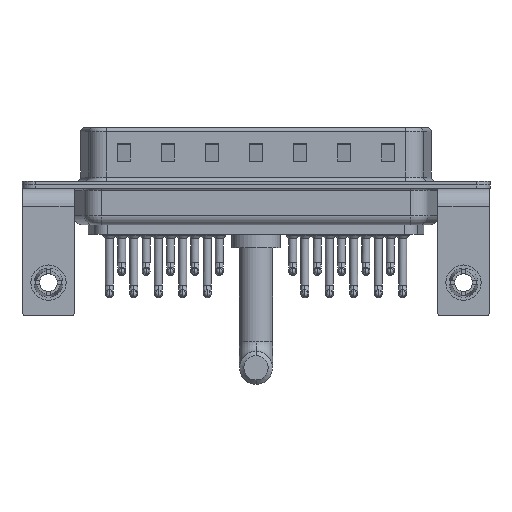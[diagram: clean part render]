
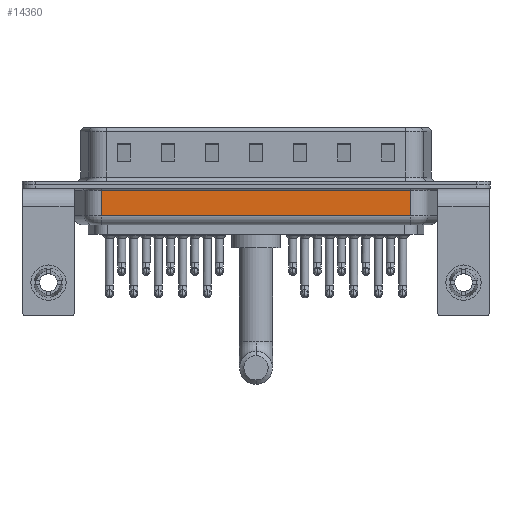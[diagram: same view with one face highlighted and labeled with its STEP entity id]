
A CAD part, front view. The second image highlights one B-rep face of the part: STEP entity #14360.
In plain terms, the highlighted planar face has unit normal (0, -1, 0).
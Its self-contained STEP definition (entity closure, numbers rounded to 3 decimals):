
#263 = DIRECTION ( 'NONE',  ( 0., 0., 1. ) ) ;
#539 = DIRECTION ( 'NONE',  ( 0., 1., 0. ) ) ;
#1984 = EDGE_CURVE ( 'NONE', #19961, #11070, #13105, .T. ) ;
#2970 = FACE_OUTER_BOUND ( 'NONE', #21036, .T. ) ;
#3172 = CARTESIAN_POINT ( 'NONE',  ( 41.044, -5.35, -4.5 ) ) ;
#3318 = ORIENTED_EDGE ( 'NONE', *, *, #22160, .F. ) ;
#5322 = CARTESIAN_POINT ( 'NONE',  ( 6.006, -5.35, -3.5 ) ) ;
#6538 = CARTESIAN_POINT ( 'NONE',  ( 6.006, -5.35, -0.65 ) ) ;
#7331 = AXIS2_PLACEMENT_3D ( 'NONE', #26988, #539, #18398 ) ;
#8326 = VERTEX_POINT ( 'NONE', #15639 ) ;
#9481 = VECTOR ( 'NONE', #27621, 1000. ) ;
#9636 = VECTOR ( 'NONE', #18620, 1000. ) ;
#11070 = VERTEX_POINT ( 'NONE', #15851 ) ;
#11337 = VECTOR ( 'NONE', #28274, 1000. ) ;
#11680 = PLANE ( 'NONE',  #7331 ) ;
#12934 = VECTOR ( 'NONE', #263, 1000. ) ;
#13105 = LINE ( 'NONE', #6538, #11337 ) ;
#13452 = VERTEX_POINT ( 'NONE', #23083 ) ;
#14360 = ADVANCED_FACE ( 'NONE', ( #2970 ), #11680, .F. ) ;
#14812 = ORIENTED_EDGE ( 'NONE', *, *, #28248, .T. ) ;
#14814 = EDGE_CURVE ( 'NONE', #13452, #8326, #16474, .T. ) ;
#15639 = CARTESIAN_POINT ( 'NONE',  ( 41.044, -5.35, -3.5 ) ) ;
#15851 = CARTESIAN_POINT ( 'NONE',  ( 6.006, -5.35, -0.65 ) ) ;
#16474 = LINE ( 'NONE', #5322, #9636 ) ;
#18398 = DIRECTION ( 'NONE',  ( 0., 0., 1. ) ) ;
#18620 = DIRECTION ( 'NONE',  ( 1., 0., 0. ) ) ;
#19139 = ORIENTED_EDGE ( 'NONE', *, *, #1984, .T. ) ;
#19230 = ORIENTED_EDGE ( 'NONE', *, *, #14814, .T. ) ;
#19961 = VERTEX_POINT ( 'NONE', #22029 ) ;
#20129 = CARTESIAN_POINT ( 'NONE',  ( 6.006, -5.35, -4.5 ) ) ;
#21036 = EDGE_LOOP ( 'NONE', ( #3318, #19230, #14812, #19139 ) ) ;
#21847 = LINE ( 'NONE', #20129, #12934 ) ;
#22029 = CARTESIAN_POINT ( 'NONE',  ( 41.044, -5.35, -0.65 ) ) ;
#22160 = EDGE_CURVE ( 'NONE', #13452, #11070, #21847, .T. ) ;
#23083 = CARTESIAN_POINT ( 'NONE',  ( 6.006, -5.35, -3.5 ) ) ;
#25466 = LINE ( 'NONE', #3172, #9481 ) ;
#26988 = CARTESIAN_POINT ( 'NONE',  ( 6.006, -5.35, -4.5 ) ) ;
#27621 = DIRECTION ( 'NONE',  ( 0., 0., 1. ) ) ;
#28248 = EDGE_CURVE ( 'NONE', #8326, #19961, #25466, .T. ) ;
#28274 = DIRECTION ( 'NONE',  ( -1., 0., 0. ) ) ;
